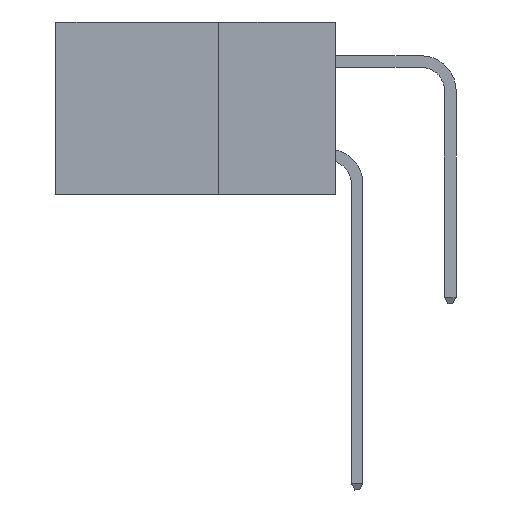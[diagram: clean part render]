
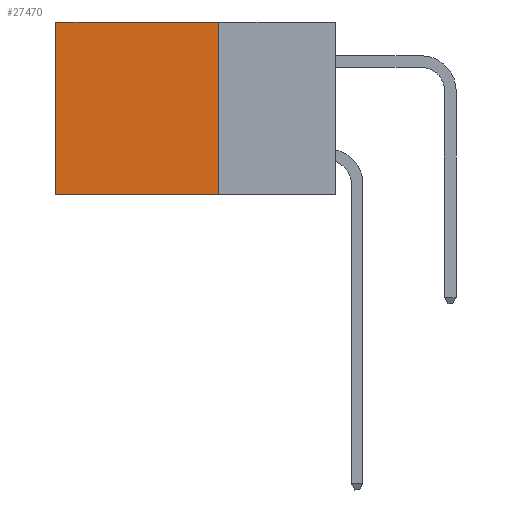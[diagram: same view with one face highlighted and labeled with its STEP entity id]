
A CAD part, left-side view. The second image highlights one B-rep face of the part: STEP entity #27470.
In plain terms, the highlighted planar face has unit normal (-1, 0, 0).
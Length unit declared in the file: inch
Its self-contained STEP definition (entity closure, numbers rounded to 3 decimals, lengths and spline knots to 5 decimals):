
#573 = VERTEX_POINT ( 'NONE', #8709 ) ;
#986 = EDGE_CURVE ( 'NONE', #573, #5292, #20749, .T. ) ;
#1996 = ORIENTED_EDGE ( 'NONE', *, *, #986, .F. ) ;
#4667 = VERTEX_POINT ( 'NONE', #10231 ) ;
#5292 = VERTEX_POINT ( 'NONE', #31207 ) ;
#6281 = FACE_OUTER_BOUND ( 'NONE', #8151, .T. ) ;
#6508 = VECTOR ( 'NONE', #10290, 39.37008 ) ;
#7008 = DIRECTION ( 'NONE',  ( 0., 0., -1. ) ) ;
#7967 = CARTESIAN_POINT ( 'NONE',  ( 0.2875, 0.25, 0. ) ) ;
#8151 = EDGE_LOOP ( 'NONE', ( #31748, #1996, #9991, #31187 ) ) ;
#8709 = CARTESIAN_POINT ( 'NONE',  ( 0.2875, 0.25, -0.37 ) ) ;
#9539 = CARTESIAN_POINT ( 'NONE',  ( 0.2875, 0.25, 0. ) ) ;
#9796 = CARTESIAN_POINT ( 'NONE',  ( 0.2875, 0.25, 0. ) ) ;
#9991 = ORIENTED_EDGE ( 'NONE', *, *, #12015, .F. ) ;
#10231 = CARTESIAN_POINT ( 'NONE',  ( 0.2875, 0.6, 0. ) ) ;
#10290 = DIRECTION ( 'NONE',  ( 0., 1., 0. ) ) ;
#10383 = VECTOR ( 'NONE', #25222, 39.37008 ) ;
#10513 = CARTESIAN_POINT ( 'NONE',  ( 0.2875, 0.25, -0.37 ) ) ;
#11785 = CARTESIAN_POINT ( 'NONE',  ( 0.2875, 0.6, 0. ) ) ;
#12015 = EDGE_CURVE ( 'NONE', #16906, #573, #24968, .T. ) ;
#12283 = LINE ( 'NONE', #11785, #34066 ) ;
#13285 = AXIS2_PLACEMENT_3D ( 'NONE', #9539, #28370, #7008 ) ;
#14502 = DIRECTION ( 'NONE',  ( 0., 0., -1. ) ) ;
#14828 = CARTESIAN_POINT ( 'NONE',  ( 0.2875, 0.25, 0. ) ) ;
#14961 = EDGE_CURVE ( 'NONE', #4667, #5292, #12283, .T. ) ;
#15140 = VECTOR ( 'NONE', #25438, 39.37008 ) ;
#16906 = VERTEX_POINT ( 'NONE', #7967 ) ;
#20749 = LINE ( 'NONE', #10513, #6508 ) ;
#24968 = LINE ( 'NONE', #14828, #10383 ) ;
#25222 = DIRECTION ( 'NONE',  ( 0., 0., -1. ) ) ;
#25438 = DIRECTION ( 'NONE',  ( 0., 1., 0. ) ) ;
#25798 = PLANE ( 'NONE',  #13285 ) ;
#27024 = EDGE_CURVE ( 'NONE', #16906, #4667, #29375, .T. ) ;
#27470 = ADVANCED_FACE ( 'NONE', ( #6281 ), #25798, .F. ) ;
#28370 = DIRECTION ( 'NONE',  ( 1., 0., 0. ) ) ;
#29375 = LINE ( 'NONE', #9796, #15140 ) ;
#31187 = ORIENTED_EDGE ( 'NONE', *, *, #27024, .T. ) ;
#31207 = CARTESIAN_POINT ( 'NONE',  ( 0.2875, 0.6, -0.37 ) ) ;
#31748 = ORIENTED_EDGE ( 'NONE', *, *, #14961, .T. ) ;
#34066 = VECTOR ( 'NONE', #14502, 39.37008 ) ;
